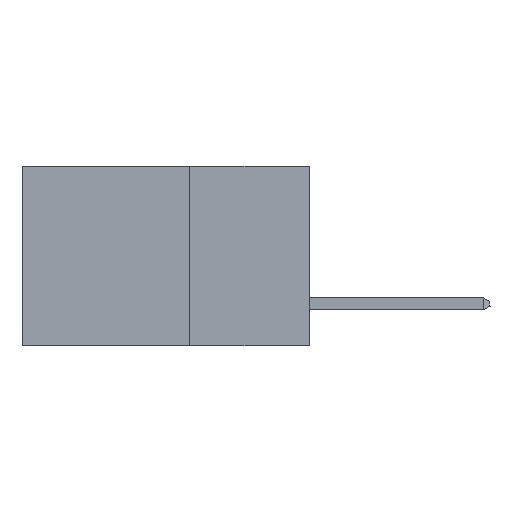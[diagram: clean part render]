
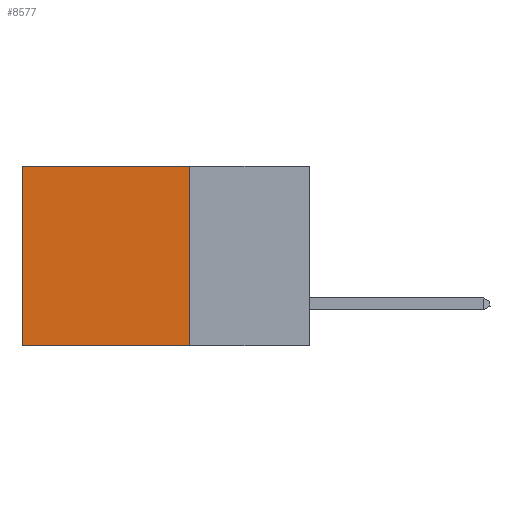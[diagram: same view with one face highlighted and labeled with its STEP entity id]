
A CAD part, left-side view. The second image highlights one B-rep face of the part: STEP entity #8577.
In plain terms, the highlighted planar face has unit normal (-1, 0, 0).
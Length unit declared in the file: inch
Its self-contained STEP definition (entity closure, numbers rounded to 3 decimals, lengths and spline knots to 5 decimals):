
#51 = ORIENTED_EDGE ( 'NONE', *, *, #1035, .T. ) ;
#539 = CARTESIAN_POINT ( 'NONE',  ( 0.2875, 0.25, -0.375 ) ) ;
#919 = DIRECTION ( 'NONE',  ( 0., 1., 0. ) ) ;
#1035 = EDGE_CURVE ( 'NONE', #5487, #10721, #2680, .T. ) ;
#1201 = CARTESIAN_POINT ( 'NONE',  ( 0.2875, 0.25, 0. ) ) ;
#1553 = DIRECTION ( 'NONE',  ( 0., 0., -1. ) ) ;
#2680 = LINE ( 'NONE', #5896, #10487 ) ;
#2750 = VECTOR ( 'NONE', #6131, 39.37008 ) ;
#3318 = ORIENTED_EDGE ( 'NONE', *, *, #8247, .F. ) ;
#3694 = ORIENTED_EDGE ( 'NONE', *, *, #11645, .T. ) ;
#4829 = VECTOR ( 'NONE', #919, 39.37008 ) ;
#5487 = VERTEX_POINT ( 'NONE', #10316 ) ;
#5896 = CARTESIAN_POINT ( 'NONE',  ( 0.2875, 0.6, -0.375 ) ) ;
#6131 = DIRECTION ( 'NONE',  ( 0., 0., -1. ) ) ;
#6352 = LINE ( 'NONE', #9785, #4829 ) ;
#6384 = EDGE_LOOP ( 'NONE', ( #51, #3318, #6745, #3694 ) ) ;
#6745 = ORIENTED_EDGE ( 'NONE', *, *, #13309, .F. ) ;
#7073 = CARTESIAN_POINT ( 'NONE',  ( 0.2875, 0.25, -0.375 ) ) ;
#8247 = EDGE_CURVE ( 'NONE', #8526, #10721, #6352, .T. ) ;
#8526 = VERTEX_POINT ( 'NONE', #539 ) ;
#8577 = ADVANCED_FACE ( 'NONE', ( #10363 ), #12611, .F. ) ;
#8915 = CARTESIAN_POINT ( 'NONE',  ( 0.2875, 0.25, 0. ) ) ;
#9630 = CARTESIAN_POINT ( 'NONE',  ( 0.2875, 0.25, -0.375 ) ) ;
#9785 = CARTESIAN_POINT ( 'NONE',  ( 0.2875, 0.25, -0.375 ) ) ;
#9998 = DIRECTION ( 'NONE',  ( 0., 1., 0. ) ) ;
#10316 = CARTESIAN_POINT ( 'NONE',  ( 0.2875, 0.6, 0. ) ) ;
#10363 = FACE_OUTER_BOUND ( 'NONE', #6384, .T. ) ;
#10487 = VECTOR ( 'NONE', #11432, 39.37008 ) ;
#10501 = VECTOR ( 'NONE', #9998, 39.37008 ) ;
#10721 = VERTEX_POINT ( 'NONE', #14254 ) ;
#11432 = DIRECTION ( 'NONE',  ( 0., 0., -1. ) ) ;
#11526 = DIRECTION ( 'NONE',  ( 1., 0., 0. ) ) ;
#11645 = EDGE_CURVE ( 'NONE', #11726, #5487, #13273, .T. ) ;
#11726 = VERTEX_POINT ( 'NONE', #1201 ) ;
#12611 = PLANE ( 'NONE',  #14117 ) ;
#13273 = LINE ( 'NONE', #8915, #10501 ) ;
#13309 = EDGE_CURVE ( 'NONE', #11726, #8526, #13913, .T. ) ;
#13913 = LINE ( 'NONE', #9630, #2750 ) ;
#14117 = AXIS2_PLACEMENT_3D ( 'NONE', #7073, #11526, #1553 ) ;
#14254 = CARTESIAN_POINT ( 'NONE',  ( 0.2875, 0.6, -0.375 ) ) ;
